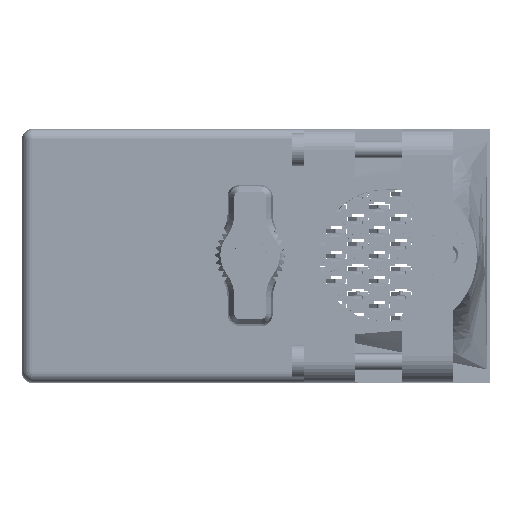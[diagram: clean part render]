
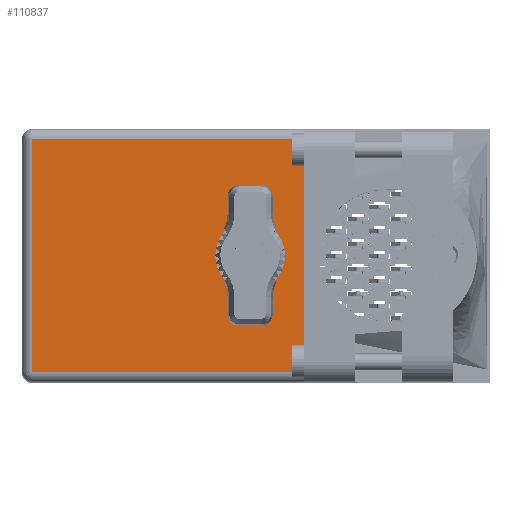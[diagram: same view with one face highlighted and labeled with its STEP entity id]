
A CAD part, top view. The second image highlights one B-rep face of the part: STEP entity #110837.
In plain terms, the highlighted face is planar.
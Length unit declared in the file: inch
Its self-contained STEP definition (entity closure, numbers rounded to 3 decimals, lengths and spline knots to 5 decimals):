
#117 = EDGE_CURVE ( 'NONE', #21465, #61144, #43189, .T. ) ;
#224 = VECTOR ( 'NONE', #91618, 39.37008 ) ;
#2795 = EDGE_CURVE ( 'NONE', #66409, #13827, #109386, .T. ) ;
#7303 = ORIENTED_EDGE ( 'NONE', *, *, #2795, .T. ) ;
#8972 = EDGE_LOOP ( 'NONE', ( #78375, #85437, #100060, #7303 ) ) ;
#13827 = VERTEX_POINT ( 'NONE', #104915 ) ;
#16394 = CARTESIAN_POINT ( 'NONE',  ( -1.3155, 1.93, 0.703 ) ) ;
#17144 = FACE_OUTER_BOUND ( 'NONE', #8972, .T. ) ;
#18122 = PLANE ( 'NONE',  #68623 ) ;
#18325 = AXIS2_PLACEMENT_3D ( 'NONE', #102928, #22721, #111082 ) ;
#21465 = VERTEX_POINT ( 'NONE', #30475 ) ;
#21929 = CARTESIAN_POINT ( 'NONE',  ( 0.3275, 1.93, -0.703 ) ) ;
#22052 = EDGE_CURVE ( 'NONE', #104724, #88615, #48004, .T. ) ;
#22721 = DIRECTION ( 'NONE',  ( 0., 1., 0. ) ) ;
#26071 = EDGE_CURVE ( 'NONE', #61144, #21465, #71662, .T. ) ;
#30475 = CARTESIAN_POINT ( 'NONE',  ( 0., 1.93, -0.17 ) ) ;
#36000 = EDGE_CURVE ( 'NONE', #13827, #104724, #109353, .T. ) ;
#36321 = EDGE_CURVE ( 'NONE', #66409, #88615, #107925, .T. ) ;
#37276 = DIRECTION ( 'NONE',  ( -1., 0., 0. ) ) ;
#43189 = CIRCLE ( 'NONE', #18325, 0.17 ) ;
#48004 = LINE ( 'NONE', #102217, #53684 ) ;
#51849 = CARTESIAN_POINT ( 'NONE',  ( 0.3275, 1.93, 0.703 ) ) ;
#53684 = VECTOR ( 'NONE', #76017, 39.37008 ) ;
#57798 = DIRECTION ( 'NONE',  ( 0., 0., 1. ) ) ;
#61144 = VERTEX_POINT ( 'NONE', #101231 ) ;
#63379 = DIRECTION ( 'NONE',  ( -1., 0., 0. ) ) ;
#63449 = FACE_BOUND ( 'NONE', #93131, .T. ) ;
#64600 = AXIS2_PLACEMENT_3D ( 'NONE', #93787, #85109, #57798 ) ;
#66409 = VERTEX_POINT ( 'NONE', #21929 ) ;
#68623 = AXIS2_PLACEMENT_3D ( 'NONE', #72153, #91247, #37276 ) ;
#71131 = ORIENTED_EDGE ( 'NONE', *, *, #26071, .F. ) ;
#71593 = CARTESIAN_POINT ( 'NONE',  ( -1.3775, 1.93, -0.703 ) ) ;
#71662 = CIRCLE ( 'NONE', #64600, 0.17 ) ;
#72153 = CARTESIAN_POINT ( 'NONE',  ( -1.3775, 1.93, -0.765 ) ) ;
#72750 = CARTESIAN_POINT ( 'NONE',  ( 0.3275, 1.93, -0.765 ) ) ;
#76017 = DIRECTION ( 'NONE',  ( 1., 0., 0. ) ) ;
#78375 = ORIENTED_EDGE ( 'NONE', *, *, #36000, .T. ) ;
#78599 = VECTOR ( 'NONE', #81712, 39.37008 ) ;
#80062 = VECTOR ( 'NONE', #63379, 39.37008 ) ;
#81712 = DIRECTION ( 'NONE',  ( 0., 0., 1. ) ) ;
#85109 = DIRECTION ( 'NONE',  ( 0., 1., 0. ) ) ;
#85437 = ORIENTED_EDGE ( 'NONE', *, *, #22052, .T. ) ;
#88615 = VERTEX_POINT ( 'NONE', #51849 ) ;
#91247 = DIRECTION ( 'NONE',  ( 0., 1., 0. ) ) ;
#91618 = DIRECTION ( 'NONE',  ( 0., 0., 1. ) ) ;
#93131 = EDGE_LOOP ( 'NONE', ( #71131, #102294 ) ) ;
#93787 = CARTESIAN_POINT ( 'NONE',  ( 0., 1.93, 0. ) ) ;
#100060 = ORIENTED_EDGE ( 'NONE', *, *, #36321, .F. ) ;
#101231 = CARTESIAN_POINT ( 'NONE',  ( 0., 1.93, 0.17 ) ) ;
#102217 = CARTESIAN_POINT ( 'NONE',  ( 0.3275, 1.93, 0.703 ) ) ;
#102294 = ORIENTED_EDGE ( 'NONE', *, *, #117, .F. ) ;
#102928 = CARTESIAN_POINT ( 'NONE',  ( 0., 1.93, 0. ) ) ;
#104724 = VERTEX_POINT ( 'NONE', #16394 ) ;
#104915 = CARTESIAN_POINT ( 'NONE',  ( -1.3155, 1.93, -0.703 ) ) ;
#107925 = LINE ( 'NONE', #72750, #78599 ) ;
#109353 = LINE ( 'NONE', #109927, #224 ) ;
#109386 = LINE ( 'NONE', #71593, #80062 ) ;
#109927 = CARTESIAN_POINT ( 'NONE',  ( -1.3155, 1.93, -0.765 ) ) ;
#110837 = ADVANCED_FACE ( 'NONE', ( #17144, #63449 ), #18122, .T. ) ;
#111082 = DIRECTION ( 'NONE',  ( 0., 0., 1. ) ) ;
